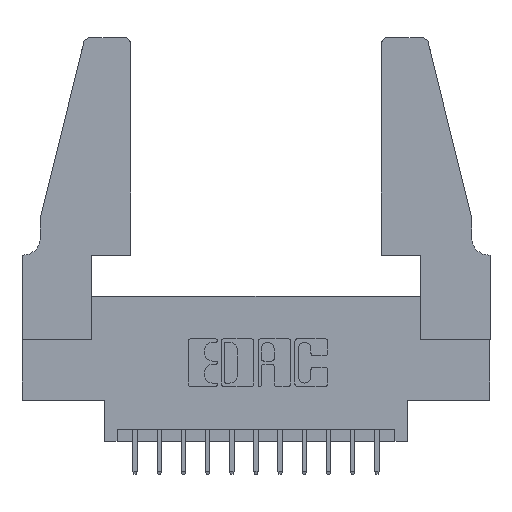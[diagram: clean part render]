
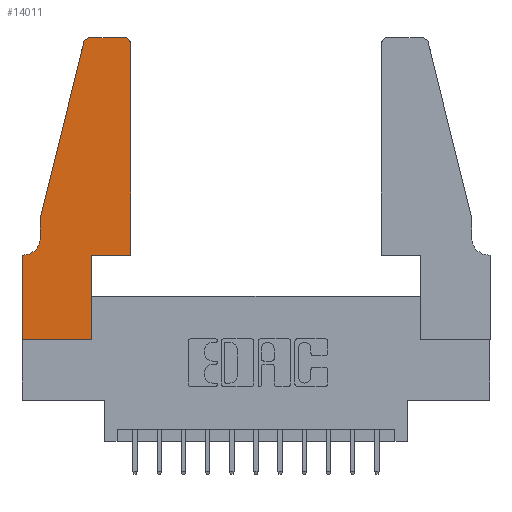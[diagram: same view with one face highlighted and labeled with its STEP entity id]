
A CAD part, top view. The second image highlights one B-rep face of the part: STEP entity #14011.
In plain terms, the highlighted planar face has unit normal (0, 0, 1).
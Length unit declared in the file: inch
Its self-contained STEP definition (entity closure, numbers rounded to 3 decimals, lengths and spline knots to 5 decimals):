
#50 = VECTOR ( 'NONE', #12454, 39.37008 ) ;
#56 = DIRECTION ( 'NONE',  ( 0., 0., -1. ) ) ;
#355 = EDGE_CURVE ( 'NONE', #14716, #3290, #8904, .T. ) ;
#409 = EDGE_CURVE ( 'NONE', #2726, #10659, #8209, .T. ) ;
#472 = CARTESIAN_POINT ( 'NONE',  ( 0.284, 1.25, 0.37 ) ) ;
#521 = CARTESIAN_POINT ( 'NONE',  ( 0.2865, 0.35, 0.37 ) ) ;
#552 = PLANE ( 'NONE',  #2124 ) ;
#802 = AXIS2_PLACEMENT_3D ( 'NONE', #13146, #56, #11841 ) ;
#1012 = CARTESIAN_POINT ( 'NONE',  ( 0.4505, 0.35, 0.37 ) ) ;
#1215 = CARTESIAN_POINT ( 'NONE',  ( 0.284, 1.22, 0.37 ) ) ;
#1301 = DIRECTION ( 'NONE',  ( 0., -1., 0. ) ) ;
#1410 = CARTESIAN_POINT ( 'NONE',  ( 0.0055, 0.35, 0.37 ) ) ;
#1476 = VERTEX_POINT ( 'NONE', #472 ) ;
#1514 = CARTESIAN_POINT ( 'NONE',  ( 0., 0., 0.37 ) ) ;
#1712 = DIRECTION ( 'NONE',  ( 0., 0., 1. ) ) ;
#1941 = CARTESIAN_POINT ( 'NONE',  ( 0., 0.35, 0.37 ) ) ;
#1954 = CARTESIAN_POINT ( 'NONE',  ( 0.4505, 0.35, 0.37 ) ) ;
#2057 = AXIS2_PLACEMENT_3D ( 'NONE', #1215, #8140, #10454 ) ;
#2124 = AXIS2_PLACEMENT_3D ( 'NONE', #1941, #1712, #13644 ) ;
#2520 = DIRECTION ( 'NONE',  ( -0.239, -0.971, 0. ) ) ;
#2639 = VERTEX_POINT ( 'NONE', #521 ) ;
#2726 = VERTEX_POINT ( 'NONE', #10228 ) ;
#2899 = ORIENTED_EDGE ( 'NONE', *, *, #8342, .T. ) ;
#3087 = VERTEX_POINT ( 'NONE', #1954 ) ;
#3262 = VECTOR ( 'NONE', #2520, 39.37008 ) ;
#3290 = VERTEX_POINT ( 'NONE', #1410 ) ;
#3632 = ORIENTED_EDGE ( 'NONE', *, *, #409, .T. ) ;
#3773 = CARTESIAN_POINT ( 'NONE',  ( 0.2865, 0.35, 0.37 ) ) ;
#3889 = DIRECTION ( 'NONE',  ( -1., 0., 0. ) ) ;
#3931 = ORIENTED_EDGE ( 'NONE', *, *, #3982, .T. ) ;
#3982 = EDGE_CURVE ( 'NONE', #4176, #11645, #8246, .T. ) ;
#4176 = VERTEX_POINT ( 'NONE', #12340 ) ;
#4371 = VERTEX_POINT ( 'NONE', #5223 ) ;
#4664 = ORIENTED_EDGE ( 'NONE', *, *, #9697, .T. ) ;
#4994 = CARTESIAN_POINT ( 'NONE',  ( 0., 0., 0.37 ) ) ;
#5150 = CARTESIAN_POINT ( 'NONE',  ( 0.0755, 0.42, 0.37 ) ) ;
#5196 = VERTEX_POINT ( 'NONE', #12421 ) ;
#5204 = LINE ( 'NONE', #14507, #7055 ) ;
#5223 = CARTESIAN_POINT ( 'NONE',  ( 0.2865, 0., 0.37 ) ) ;
#5309 = ORIENTED_EDGE ( 'NONE', *, *, #11540, .T. ) ;
#5748 = ORIENTED_EDGE ( 'NONE', *, *, #7136, .T. ) ;
#5850 = ORIENTED_EDGE ( 'NONE', *, *, #5973, .T. ) ;
#5959 = ORIENTED_EDGE ( 'NONE', *, *, #355, .T. ) ;
#5973 = EDGE_CURVE ( 'NONE', #5196, #9966, #7313, .T. ) ;
#6077 = CARTESIAN_POINT ( 'NONE',  ( 0.4205, 1.22, 0.37 ) ) ;
#6103 = DIRECTION ( 'NONE',  ( 0., 1., 0. ) ) ;
#6200 = CARTESIAN_POINT ( 'NONE',  ( 0.4505, 0.35, 0.37 ) ) ;
#6601 = LINE ( 'NONE', #9049, #50 ) ;
#7055 = VECTOR ( 'NONE', #3889, 39.37008 ) ;
#7092 = DIRECTION ( 'NONE',  ( 0., 0., 1. ) ) ;
#7136 = EDGE_CURVE ( 'NONE', #2639, #3087, #9819, .T. ) ;
#7178 = ORIENTED_EDGE ( 'NONE', *, *, #8789, .T. ) ;
#7313 = CIRCLE ( 'NONE', #12995, 0.03 ) ;
#7580 = DIRECTION ( 'NONE',  ( 1., 0., 0. ) ) ;
#8140 = DIRECTION ( 'NONE',  ( 0., 0., 1. ) ) ;
#8209 = LINE ( 'NONE', #11770, #3262 ) ;
#8246 = LINE ( 'NONE', #14091, #8513 ) ;
#8342 = EDGE_CURVE ( 'NONE', #10659, #14716, #8372, .T. ) ;
#8372 = LINE ( 'NONE', #14064, #15013 ) ;
#8513 = VECTOR ( 'NONE', #10621, 39.37008 ) ;
#8789 = EDGE_CURVE ( 'NONE', #3290, #4176, #6601, .T. ) ;
#8904 = CIRCLE ( 'NONE', #802, 0.07 ) ;
#8986 = EDGE_CURVE ( 'NONE', #4371, #2639, #14093, .T. ) ;
#9049 = CARTESIAN_POINT ( 'NONE',  ( 0.0755, 0.35, 0.37 ) ) ;
#9432 = VECTOR ( 'NONE', #12243, 39.37008 ) ;
#9697 = EDGE_CURVE ( 'NONE', #3087, #5196, #11346, .T. ) ;
#9819 = LINE ( 'NONE', #6200, #13013 ) ;
#9966 = VERTEX_POINT ( 'NONE', #10238 ) ;
#10110 = ORIENTED_EDGE ( 'NONE', *, *, #14801, .T. ) ;
#10155 = VECTOR ( 'NONE', #13714, 39.37008 ) ;
#10228 = CARTESIAN_POINT ( 'NONE',  ( 0.25487, 1.22718, 0.37 ) ) ;
#10238 = CARTESIAN_POINT ( 'NONE',  ( 0.4205, 1.25, 0.37 ) ) ;
#10454 = DIRECTION ( 'NONE',  ( 1., 0., 0. ) ) ;
#10621 = DIRECTION ( 'NONE',  ( 0., -1., 0. ) ) ;
#10659 = VERTEX_POINT ( 'NONE', #12823 ) ;
#10769 = DIRECTION ( 'NONE',  ( 1., 0., 0. ) ) ;
#10838 = LINE ( 'NONE', #1514, #9432 ) ;
#11029 = ORIENTED_EDGE ( 'NONE', *, *, #8986, .T. ) ;
#11346 = LINE ( 'NONE', #1012, #10155 ) ;
#11405 = CIRCLE ( 'NONE', #2057, 0.03 ) ;
#11540 = EDGE_CURVE ( 'NONE', #1476, #2726, #11405, .T. ) ;
#11571 = EDGE_CURVE ( 'NONE', #11645, #4371, #10838, .T. ) ;
#11645 = VERTEX_POINT ( 'NONE', #4994 ) ;
#11770 = CARTESIAN_POINT ( 'NONE',  ( 0.0755, 0.5, 0.37 ) ) ;
#11841 = DIRECTION ( 'NONE',  ( -1., 0., 0. ) ) ;
#12035 = ORIENTED_EDGE ( 'NONE', *, *, #11571, .T. ) ;
#12210 = FACE_OUTER_BOUND ( 'NONE', #14278, .T. ) ;
#12243 = DIRECTION ( 'NONE',  ( 1., 0., 0. ) ) ;
#12340 = CARTESIAN_POINT ( 'NONE',  ( 0., 0.35, 0.37 ) ) ;
#12421 = CARTESIAN_POINT ( 'NONE',  ( 0.4505, 1.22, 0.37 ) ) ;
#12454 = DIRECTION ( 'NONE',  ( -1., 0., 0. ) ) ;
#12823 = CARTESIAN_POINT ( 'NONE',  ( 0.0755, 0.5, 0.37 ) ) ;
#12995 = AXIS2_PLACEMENT_3D ( 'NONE', #6077, #7092, #10769 ) ;
#13013 = VECTOR ( 'NONE', #7580, 39.37008 ) ;
#13146 = CARTESIAN_POINT ( 'NONE',  ( 0.0055, 0.42, 0.37 ) ) ;
#13644 = DIRECTION ( 'NONE',  ( 1., 0., 0. ) ) ;
#13714 = DIRECTION ( 'NONE',  ( 0., 1., 0. ) ) ;
#14011 = ADVANCED_FACE ( 'NONE', ( #12210 ), #552, .T. ) ;
#14064 = CARTESIAN_POINT ( 'NONE',  ( 0.0755, 0.5, 0.37 ) ) ;
#14091 = CARTESIAN_POINT ( 'NONE',  ( 0., 0., 0.37 ) ) ;
#14093 = LINE ( 'NONE', #3773, #14558 ) ;
#14278 = EDGE_LOOP ( 'NONE', ( #10110, #5309, #3632, #2899, #5959, #7178, #3931, #12035, #11029, #5748, #4664, #5850 ) ) ;
#14507 = CARTESIAN_POINT ( 'NONE',  ( 0.2605, 1.25, 0.37 ) ) ;
#14558 = VECTOR ( 'NONE', #6103, 39.37008 ) ;
#14716 = VERTEX_POINT ( 'NONE', #5150 ) ;
#14801 = EDGE_CURVE ( 'NONE', #9966, #1476, #5204, .T. ) ;
#15013 = VECTOR ( 'NONE', #1301, 39.37008 ) ;
